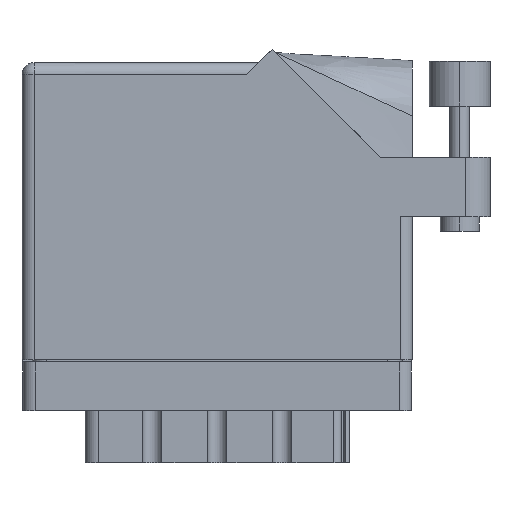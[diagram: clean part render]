
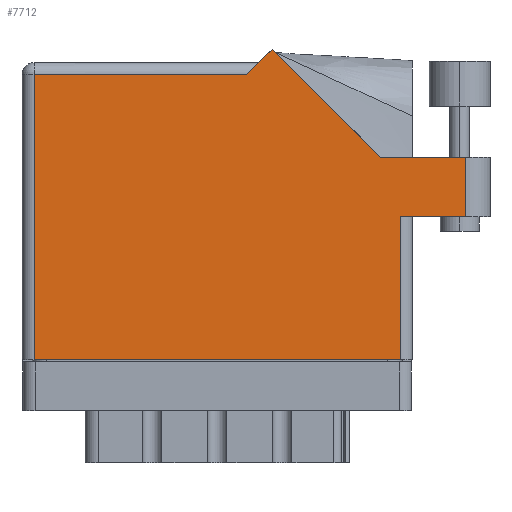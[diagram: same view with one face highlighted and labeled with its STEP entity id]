
A CAD part, front view. The second image highlights one B-rep face of the part: STEP entity #7712.
In plain terms, the highlighted face is planar.
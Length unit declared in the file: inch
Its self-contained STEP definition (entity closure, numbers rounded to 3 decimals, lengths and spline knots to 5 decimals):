
#421 = DIRECTION ( 'NONE',  ( -1., 0., 0. ) ) ;
#850 = VERTEX_POINT ( 'NONE', #28723 ) ;
#2290 = VERTEX_POINT ( 'NONE', #33686 ) ;
#2817 = VECTOR ( 'NONE', #11743, 39.37008 ) ;
#2912 = DIRECTION ( 'NONE',  ( 0., 0., -1. ) ) ;
#4016 = CARTESIAN_POINT ( 'NONE',  ( 2.285, 1.044, 0. ) ) ;
#4142 = ORIENTED_EDGE ( 'NONE', *, *, #21895, .T. ) ;
#4193 = CARTESIAN_POINT ( 'NONE',  ( 0.062, 1.468, 0. ) ) ;
#4280 = VECTOR ( 'NONE', #8350, 39.37008 ) ;
#4706 = LINE ( 'NONE', #5602, #4280 ) ;
#5098 = VECTOR ( 'NONE', #12638, 39.37008 ) ;
#5602 = CARTESIAN_POINT ( 'NONE',  ( 0.062, 0., 0. ) ) ;
#6616 = CARTESIAN_POINT ( 'NONE',  ( 0., 1.468, 0. ) ) ;
#7222 = ORIENTED_EDGE ( 'NONE', *, *, #21271, .T. ) ;
#7712 = ADVANCED_FACE ( 'NONE', ( #16636 ), #11682, .F. ) ;
#8273 = CARTESIAN_POINT ( 'NONE',  ( 1.948, 0.737, 0. ) ) ;
#8350 = DIRECTION ( 'NONE',  ( 0., -1., 0. ) ) ;
#8392 = ORIENTED_EDGE ( 'NONE', *, *, #27474, .T. ) ;
#8460 = VERTEX_POINT ( 'NONE', #8892 ) ;
#8892 = CARTESIAN_POINT ( 'NONE',  ( 1.155, 1.468, 0. ) ) ;
#9211 = DIRECTION ( 'NONE',  ( 1., 0., 0. ) ) ;
#9613 = VERTEX_POINT ( 'NONE', #4193 ) ;
#9706 = LINE ( 'NONE', #8273, #19552 ) ;
#10692 = VECTOR ( 'NONE', #36275, 39.37008 ) ;
#11584 = LINE ( 'NONE', #16209, #26406 ) ;
#11682 = PLANE ( 'NONE',  #26189 ) ;
#11743 = DIRECTION ( 'NONE',  ( -0.707, -0.707, 0. ) ) ;
#11761 = EDGE_CURVE ( 'NONE', #36521, #17266, #14712, .T. ) ;
#12558 = CARTESIAN_POINT ( 'NONE',  ( 1.948, 0., 0. ) ) ;
#12638 = DIRECTION ( 'NONE',  ( -1., 0., 0. ) ) ;
#13283 = CARTESIAN_POINT ( 'NONE',  ( 1.84442, 1.044, 0. ) ) ;
#14184 = EDGE_CURVE ( 'NONE', #9613, #34843, #4706, .T. ) ;
#14565 = ORIENTED_EDGE ( 'NONE', *, *, #36869, .T. ) ;
#14712 = LINE ( 'NONE', #33645, #10692 ) ;
#15095 = LINE ( 'NONE', #21018, #19555 ) ;
#16209 = CARTESIAN_POINT ( 'NONE',  ( 2.285, 1.044, 0. ) ) ;
#16636 = FACE_OUTER_BOUND ( 'NONE', #21465, .T. ) ;
#17266 = VERTEX_POINT ( 'NONE', #21768 ) ;
#18220 = ORIENTED_EDGE ( 'NONE', *, *, #26179, .T. ) ;
#18807 = DIRECTION ( 'NONE',  ( 0., 1., 0. ) ) ;
#19032 = DIRECTION ( 'NONE',  ( -0.707, 0.707, 0. ) ) ;
#19552 = VECTOR ( 'NONE', #31253, 39.37008 ) ;
#19555 = VECTOR ( 'NONE', #9211, 39.37008 ) ;
#19717 = ORIENTED_EDGE ( 'NONE', *, *, #23473, .T. ) ;
#19960 = LINE ( 'NONE', #24652, #27645 ) ;
#21018 = CARTESIAN_POINT ( 'NONE',  ( 0., 0., 0. ) ) ;
#21271 = EDGE_CURVE ( 'NONE', #2290, #850, #28165, .T. ) ;
#21465 = EDGE_LOOP ( 'NONE', ( #25052, #21794, #4142, #7222, #19717, #8392, #23278, #18220, #14565 ) ) ;
#21768 = CARTESIAN_POINT ( 'NONE',  ( 2.285, 0.737, 0. ) ) ;
#21794 = ORIENTED_EDGE ( 'NONE', *, *, #25185, .T. ) ;
#21895 = EDGE_CURVE ( 'NONE', #27444, #2290, #19960, .T. ) ;
#22129 = LINE ( 'NONE', #29191, #2817 ) ;
#23101 = CARTESIAN_POINT ( 'NONE',  ( 0., 1.53, 0. ) ) ;
#23278 = ORIENTED_EDGE ( 'NONE', *, *, #14184, .T. ) ;
#23473 = EDGE_CURVE ( 'NONE', #850, #8460, #22129, .T. ) ;
#24652 = CARTESIAN_POINT ( 'NONE',  ( 2.41, 1.044, 0. ) ) ;
#25052 = ORIENTED_EDGE ( 'NONE', *, *, #11761, .T. ) ;
#25185 = EDGE_CURVE ( 'NONE', #17266, #27444, #11584, .T. ) ;
#26179 = EDGE_CURVE ( 'NONE', #34843, #35098, #15095, .T. ) ;
#26189 = AXIS2_PLACEMENT_3D ( 'NONE', #23101, #2912, #421 ) ;
#26380 = VECTOR ( 'NONE', #19032, 39.37008 ) ;
#26406 = VECTOR ( 'NONE', #18807, 39.37008 ) ;
#27444 = VERTEX_POINT ( 'NONE', #4016 ) ;
#27474 = EDGE_CURVE ( 'NONE', #8460, #9613, #35580, .T. ) ;
#27645 = VECTOR ( 'NONE', #36160, 39.37008 ) ;
#28165 = LINE ( 'NONE', #13283, #26380 ) ;
#28723 = CARTESIAN_POINT ( 'NONE',  ( 1.28771, 1.60071, 0. ) ) ;
#29191 = CARTESIAN_POINT ( 'NONE',  ( 1.217, 1.53, 0. ) ) ;
#31253 = DIRECTION ( 'NONE',  ( 0., 1., 0. ) ) ;
#32253 = CARTESIAN_POINT ( 'NONE',  ( 0.062, 0., 0. ) ) ;
#33645 = CARTESIAN_POINT ( 'NONE',  ( 2.01, 0.737, 0. ) ) ;
#33686 = CARTESIAN_POINT ( 'NONE',  ( 1.84442, 1.044, 0. ) ) ;
#34843 = VERTEX_POINT ( 'NONE', #32253 ) ;
#34904 = CARTESIAN_POINT ( 'NONE',  ( 1.948, 0.737, 0. ) ) ;
#35098 = VERTEX_POINT ( 'NONE', #12558 ) ;
#35580 = LINE ( 'NONE', #6616, #5098 ) ;
#36160 = DIRECTION ( 'NONE',  ( -1., 0., 0. ) ) ;
#36275 = DIRECTION ( 'NONE',  ( 1., 0., 0. ) ) ;
#36521 = VERTEX_POINT ( 'NONE', #34904 ) ;
#36869 = EDGE_CURVE ( 'NONE', #35098, #36521, #9706, .T. ) ;
